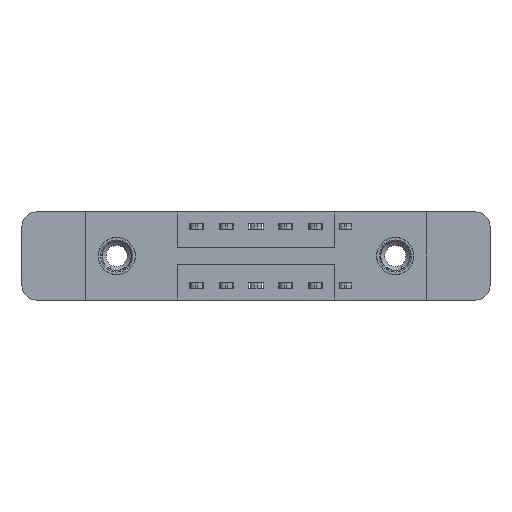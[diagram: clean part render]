
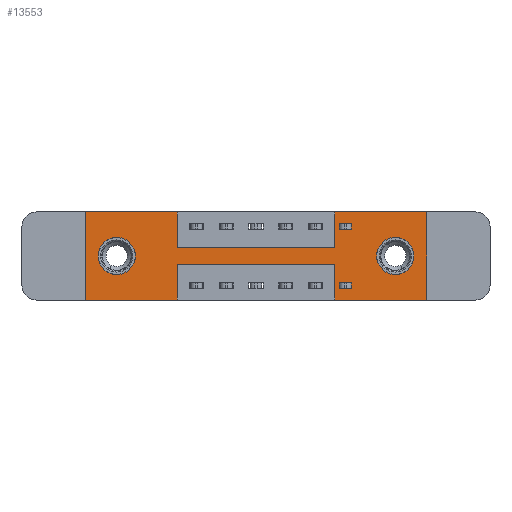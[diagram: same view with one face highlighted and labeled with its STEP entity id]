
A CAD part, front view. The second image highlights one B-rep face of the part: STEP entity #13553.
In plain terms, the highlighted planar face has unit normal (0, -1, 0).
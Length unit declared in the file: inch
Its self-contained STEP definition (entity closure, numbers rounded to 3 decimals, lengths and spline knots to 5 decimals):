
#25 = DIRECTION ( 'NONE',  ( 0., 0., -1. ) ) ;
#91 = VECTOR ( 'NONE', #4444, 39.37008 ) ;
#150 = VERTEX_POINT ( 'NONE', #9284 ) ;
#261 = VERTEX_POINT ( 'NONE', #13345 ) ;
#399 = ORIENTED_EDGE ( 'NONE', *, *, #5519, .F. ) ;
#565 = VERTEX_POINT ( 'NONE', #4382 ) ;
#577 = CARTESIAN_POINT ( 'NONE',  ( 0., 0., -0.37 ) ) ;
#695 = EDGE_CURVE ( 'NONE', #565, #1605, #10885, .T. ) ;
#753 = DIRECTION ( 'NONE',  ( -1., 0., 0. ) ) ;
#849 = CARTESIAN_POINT ( 'NONE',  ( 0., 0., -0.37 ) ) ;
#926 = DIRECTION ( 'NONE',  ( -1., 0., 0. ) ) ;
#1163 = LINE ( 'NONE', #7562, #12177 ) ;
#1268 = CARTESIAN_POINT ( 'NONE',  ( 0.1325, 0., -0.263 ) ) ;
#1305 = VECTOR ( 'NONE', #753, 39.37008 ) ;
#1605 = VERTEX_POINT ( 'NONE', #8044 ) ;
#1636 = EDGE_CURVE ( 'NONE', #261, #4367, #10090, .T. ) ;
#1660 = DIRECTION ( 'NONE',  ( 0., 0., 1. ) ) ;
#1689 = LINE ( 'NONE', #577, #12127 ) ;
#1766 = ORIENTED_EDGE ( 'NONE', *, *, #2574, .F. ) ;
#1819 = ORIENTED_EDGE ( 'NONE', *, *, #695, .F. ) ;
#1879 = VERTEX_POINT ( 'NONE', #2421 ) ;
#1888 = LINE ( 'NONE', #3020, #1305 ) ;
#1909 = DIRECTION ( 'NONE',  ( 0., -1., 0. ) ) ;
#1939 = CARTESIAN_POINT ( 'NONE',  ( 0.3875, 0., -0.15 ) ) ;
#2015 = CARTESIAN_POINT ( 'NONE',  ( 0.3875, 0., 0. ) ) ;
#2024 = AXIS2_PLACEMENT_3D ( 'NONE', #8194, #13531, #25 ) ;
#2025 = VERTEX_POINT ( 'NONE', #1268 ) ;
#2252 = VERTEX_POINT ( 'NONE', #3640 ) ;
#2302 = CIRCLE ( 'NONE', #9690, 0.078 ) ;
#2354 = VERTEX_POINT ( 'NONE', #3066 ) ;
#2421 = CARTESIAN_POINT ( 'NONE',  ( 1.3025, 0., -0.263 ) ) ;
#2524 = EDGE_CURVE ( 'NONE', #2252, #3796, #9668, .T. ) ;
#2574 = EDGE_CURVE ( 'NONE', #2354, #3833, #8881, .T. ) ;
#2647 = CARTESIAN_POINT ( 'NONE',  ( 0.3875, 0., -0.37 ) ) ;
#2651 = DIRECTION ( 'NONE',  ( 0., 0., 1. ) ) ;
#2718 = LINE ( 'NONE', #2647, #12281 ) ;
#2794 = CARTESIAN_POINT ( 'NONE',  ( 0., 0., 0. ) ) ;
#3020 = CARTESIAN_POINT ( 'NONE',  ( 0.3875, 0., -0.22 ) ) ;
#3066 = CARTESIAN_POINT ( 'NONE',  ( 1.0475, 0., -0.15 ) ) ;
#3290 = CARTESIAN_POINT ( 'NONE',  ( 1.435, 0., -0.37 ) ) ;
#3566 = CARTESIAN_POINT ( 'NONE',  ( 1.0475, 0., 0. ) ) ;
#3640 = CARTESIAN_POINT ( 'NONE',  ( 1.435, 0., 0. ) ) ;
#3777 = ORIENTED_EDGE ( 'NONE', *, *, #5286, .F. ) ;
#3796 = VERTEX_POINT ( 'NONE', #3290 ) ;
#3833 = VERTEX_POINT ( 'NONE', #8671 ) ;
#3938 = DIRECTION ( 'NONE',  ( -1., 0., 0. ) ) ;
#4181 = DIRECTION ( 'NONE',  ( 1., 0., 0. ) ) ;
#4233 = VECTOR ( 'NONE', #11778, 39.37008 ) ;
#4367 = VERTEX_POINT ( 'NONE', #5941 ) ;
#4382 = CARTESIAN_POINT ( 'NONE',  ( 1.0475, 0., -0.37 ) ) ;
#4404 = ORIENTED_EDGE ( 'NONE', *, *, #1636, .F. ) ;
#4414 = DIRECTION ( 'NONE',  ( 1., 0., 0. ) ) ;
#4444 = DIRECTION ( 'NONE',  ( 0., 0., 1. ) ) ;
#4487 = CIRCLE ( 'NONE', #12313, 0.078 ) ;
#4695 = CARTESIAN_POINT ( 'NONE',  ( 0.1325, 0., -0.185 ) ) ;
#4697 = ORIENTED_EDGE ( 'NONE', *, *, #13351, .F. ) ;
#4823 = ORIENTED_EDGE ( 'NONE', *, *, #6320, .T. ) ;
#4870 = AXIS2_PLACEMENT_3D ( 'NONE', #13688, #10545, #7114 ) ;
#5081 = CARTESIAN_POINT ( 'NONE',  ( 0., 0., -0.37 ) ) ;
#5129 = CARTESIAN_POINT ( 'NONE',  ( 1.3025, 0., -0.185 ) ) ;
#5286 = EDGE_CURVE ( 'NONE', #1605, #150, #1888, .T. ) ;
#5390 = VECTOR ( 'NONE', #926, 39.37008 ) ;
#5519 = EDGE_CURVE ( 'NONE', #150, #6454, #2718, .T. ) ;
#5529 = CARTESIAN_POINT ( 'NONE',  ( 1.435, 0., 0. ) ) ;
#5604 = EDGE_LOOP ( 'NONE', ( #399, #3777, #1819, #10462, #10392, #8427, #1766, #8458, #10551, #5972, #4404, #4697 ) ) ;
#5734 = DIRECTION ( 'NONE',  ( 0., 0., 1. ) ) ;
#5874 = AXIS2_PLACEMENT_3D ( 'NONE', #849, #1909, #13602 ) ;
#5941 = CARTESIAN_POINT ( 'NONE',  ( 0., 0., 0. ) ) ;
#5972 = ORIENTED_EDGE ( 'NONE', *, *, #8403, .F. ) ;
#6021 = CARTESIAN_POINT ( 'NONE',  ( 0., 0., 0. ) ) ;
#6089 = LINE ( 'NONE', #6021, #9038 ) ;
#6164 = CARTESIAN_POINT ( 'NONE',  ( 0.3875, 0., -0.37 ) ) ;
#6243 = VECTOR ( 'NONE', #5734, 39.37008 ) ;
#6252 = EDGE_CURVE ( 'NONE', #1879, #10221, #4487, .T. ) ;
#6320 = EDGE_CURVE ( 'NONE', #10221, #1879, #6946, .T. ) ;
#6454 = VERTEX_POINT ( 'NONE', #6164 ) ;
#6720 = EDGE_CURVE ( 'NONE', #3833, #2252, #8382, .T. ) ;
#6946 = CIRCLE ( 'NONE', #2024, 0.078 ) ;
#7091 = DIRECTION ( 'NONE',  ( 0., 0., -1. ) ) ;
#7114 = DIRECTION ( 'NONE',  ( 0., 0., 1. ) ) ;
#7225 = EDGE_CURVE ( 'NONE', #11229, #11199, #8946, .T. ) ;
#7322 = ORIENTED_EDGE ( 'NONE', *, *, #10381, .T. ) ;
#7548 = EDGE_CURVE ( 'NONE', #3796, #565, #9338, .T. ) ;
#7562 = CARTESIAN_POINT ( 'NONE',  ( 0.3875, 0., -0.15 ) ) ;
#8044 = CARTESIAN_POINT ( 'NONE',  ( 1.0475, 0., -0.22 ) ) ;
#8194 = CARTESIAN_POINT ( 'NONE',  ( 1.3025, 0., -0.185 ) ) ;
#8348 = ORIENTED_EDGE ( 'NONE', *, *, #9729, .T. ) ;
#8382 = LINE ( 'NONE', #9644, #8709 ) ;
#8403 = EDGE_CURVE ( 'NONE', #4367, #11229, #6089, .T. ) ;
#8427 = ORIENTED_EDGE ( 'NONE', *, *, #6720, .F. ) ;
#8458 = ORIENTED_EDGE ( 'NONE', *, *, #8536, .F. ) ;
#8501 = ORIENTED_EDGE ( 'NONE', *, *, #6252, .T. ) ;
#8536 = EDGE_CURVE ( 'NONE', #11199, #2354, #1163, .T. ) ;
#8561 = FACE_OUTER_BOUND ( 'NONE', #5604, .T. ) ;
#8671 = CARTESIAN_POINT ( 'NONE',  ( 1.0475, 0., 0. ) ) ;
#8709 = VECTOR ( 'NONE', #4181, 39.37008 ) ;
#8877 = CARTESIAN_POINT ( 'NONE',  ( 0.3875, 0., 0. ) ) ;
#8880 = DIRECTION ( 'NONE',  ( 0., 1., 0. ) ) ;
#8881 = LINE ( 'NONE', #3566, #9167 ) ;
#8946 = LINE ( 'NONE', #8877, #10730 ) ;
#9038 = VECTOR ( 'NONE', #11478, 39.37008 ) ;
#9106 = CIRCLE ( 'NONE', #4870, 0.078 ) ;
#9113 = DIRECTION ( 'NONE',  ( 0., 1., 0. ) ) ;
#9167 = VECTOR ( 'NONE', #2651, 39.37008 ) ;
#9284 = CARTESIAN_POINT ( 'NONE',  ( 0.3875, 0., -0.22 ) ) ;
#9338 = LINE ( 'NONE', #5081, #5390 ) ;
#9644 = CARTESIAN_POINT ( 'NONE',  ( 0., 0., 0. ) ) ;
#9668 = LINE ( 'NONE', #5529, #4233 ) ;
#9690 = AXIS2_PLACEMENT_3D ( 'NONE', #4695, #8880, #1660 ) ;
#9729 = EDGE_CURVE ( 'NONE', #10294, #2025, #2302, .T. ) ;
#10014 = DIRECTION ( 'NONE',  ( 0., 0., -1. ) ) ;
#10076 = DIRECTION ( 'NONE',  ( 0., 0., -1. ) ) ;
#10090 = LINE ( 'NONE', #2794, #6243 ) ;
#10181 = EDGE_LOOP ( 'NONE', ( #4823, #8501 ) ) ;
#10221 = VERTEX_POINT ( 'NONE', #13206 ) ;
#10294 = VERTEX_POINT ( 'NONE', #13618 ) ;
#10381 = EDGE_CURVE ( 'NONE', #2025, #10294, #9106, .T. ) ;
#10392 = ORIENTED_EDGE ( 'NONE', *, *, #2524, .F. ) ;
#10459 = PLANE ( 'NONE',  #5874 ) ;
#10462 = ORIENTED_EDGE ( 'NONE', *, *, #7548, .F. ) ;
#10545 = DIRECTION ( 'NONE',  ( 0., 1., 0. ) ) ;
#10551 = ORIENTED_EDGE ( 'NONE', *, *, #7225, .F. ) ;
#10730 = VECTOR ( 'NONE', #10076, 39.37008 ) ;
#10885 = LINE ( 'NONE', #11091, #91 ) ;
#11091 = CARTESIAN_POINT ( 'NONE',  ( 1.0475, 0., -0.37 ) ) ;
#11199 = VERTEX_POINT ( 'NONE', #1939 ) ;
#11229 = VERTEX_POINT ( 'NONE', #2015 ) ;
#11478 = DIRECTION ( 'NONE',  ( 1., 0., 0. ) ) ;
#11505 = FACE_BOUND ( 'NONE', #12667, .T. ) ;
#11778 = DIRECTION ( 'NONE',  ( 0., 0., -1. ) ) ;
#12127 = VECTOR ( 'NONE', #3938, 39.37008 ) ;
#12177 = VECTOR ( 'NONE', #4414, 39.37008 ) ;
#12281 = VECTOR ( 'NONE', #10014, 39.37008 ) ;
#12313 = AXIS2_PLACEMENT_3D ( 'NONE', #5129, #9113, #7091 ) ;
#12667 = EDGE_LOOP ( 'NONE', ( #8348, #7322 ) ) ;
#12699 = FACE_BOUND ( 'NONE', #10181, .T. ) ;
#13206 = CARTESIAN_POINT ( 'NONE',  ( 1.3025, 0., -0.107 ) ) ;
#13345 = CARTESIAN_POINT ( 'NONE',  ( 0., 0., -0.37 ) ) ;
#13351 = EDGE_CURVE ( 'NONE', #6454, #261, #1689, .T. ) ;
#13531 = DIRECTION ( 'NONE',  ( 0., 1., 0. ) ) ;
#13553 = ADVANCED_FACE ( 'NONE', ( #12699, #11505, #8561 ), #10459, .T. ) ;
#13602 = DIRECTION ( 'NONE',  ( 0., 0., -1. ) ) ;
#13618 = CARTESIAN_POINT ( 'NONE',  ( 0.1325, 0., -0.107 ) ) ;
#13688 = CARTESIAN_POINT ( 'NONE',  ( 0.1325, 0., -0.185 ) ) ;
